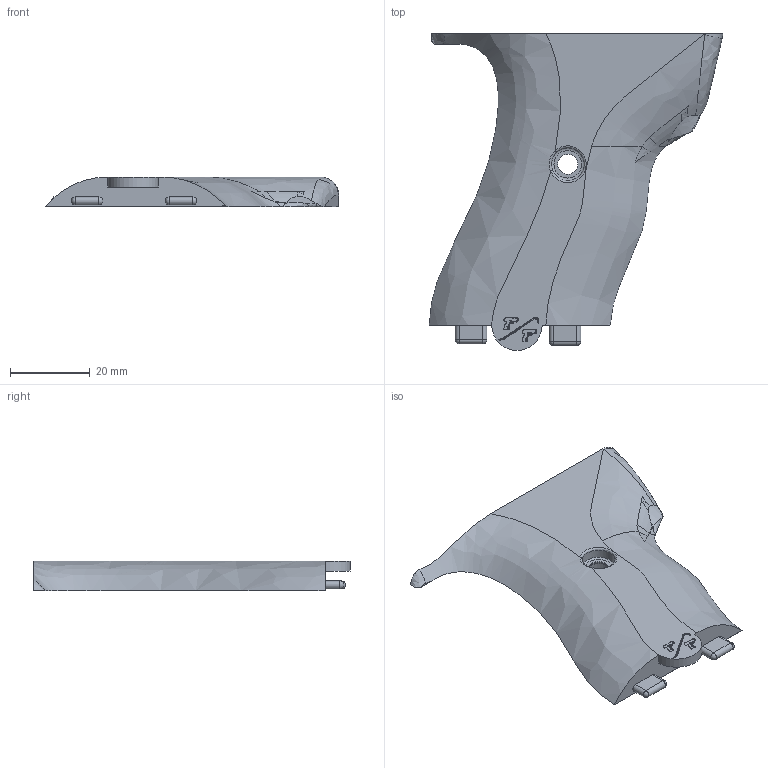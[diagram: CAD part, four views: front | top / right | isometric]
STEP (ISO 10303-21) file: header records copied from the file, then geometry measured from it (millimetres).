
FILE_DESCRIPTION(/* description */ (''),/* implementation_level */ '2;1');
FILE_NAME(/* name */ 'Freeman1337-lopoint-grip-R.step',/* time_stamp */ '2021-05-10T14:42:54-07:00',/* author */ (''),/* organization */ (''),/* preprocessor_version */ 'ST-DEVELOPER v18.1',/* originating_system */ 'Autodesk Translation Framework v10.6.0.1341',/* authorisation */ '');
FILE_SCHEMA (('AUTOMOTIVE_DESIGN { 1 0 10303 214 3 1 1 }'));
Products named in the file (1): Freeman1337-lopoint-grip-R
Bounding box: 73.56 x 79.31 x 7.5 mm (x, y, z)
Volume: 18883.7 mm3; surface area: 8894.7 mm2
Topology: 1 solids, 1 shells, 1979 faces, 5444 edges, 3623 vertices
Faces by surface type: bspline 1650, plane 306, cylinder 15, sphere 4, torus 4
Full cylindrical faces by diameter (mm): 5 x1, 8.2 x2
Entity records: 68579 total; most frequent: CARTESIAN_POINT 34543, ORIENTED_EDGE 10884, EDGE_CURVE 5442, VERTEX_POINT 3624, DIRECTION 2820, EDGE_LOOP 2140, LINE 2078, VECTOR 2078
